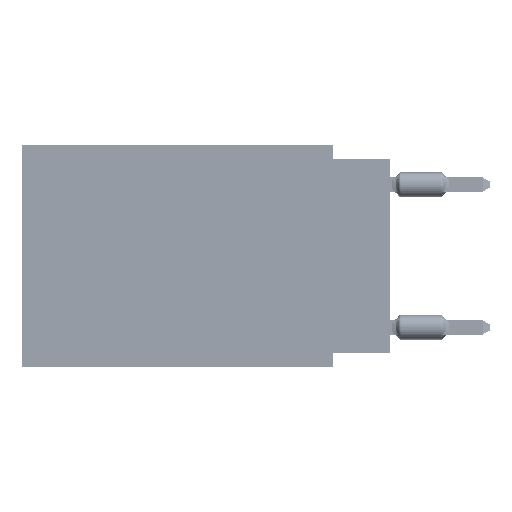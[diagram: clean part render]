
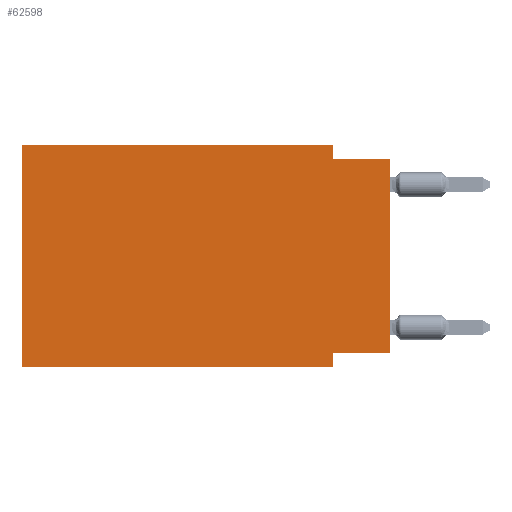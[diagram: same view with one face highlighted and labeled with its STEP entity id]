
A CAD part, left-side view. The second image highlights one B-rep face of the part: STEP entity #62598.
In plain terms, the highlighted planar face has unit normal (-1, 0, 0).
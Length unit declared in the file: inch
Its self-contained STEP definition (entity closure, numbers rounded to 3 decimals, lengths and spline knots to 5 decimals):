
#999 = LINE ( 'NONE', #45728, #61060 ) ;
#1266 = VERTEX_POINT ( 'NONE', #63140 ) ;
#2032 = PLANE ( 'NONE',  #42727 ) ;
#4770 = CARTESIAN_POINT ( 'NONE',  ( 0., 0., -0.365 ) ) ;
#6978 = CARTESIAN_POINT ( 'NONE',  ( 0., 0.1, 0. ) ) ;
#9306 = CARTESIAN_POINT ( 'NONE',  ( 0., 0.1, 0. ) ) ;
#11625 = EDGE_CURVE ( 'NONE', #47348, #21724, #61933, .T. ) ;
#12854 = CARTESIAN_POINT ( 'NONE',  ( 0., 0.645, 0. ) ) ;
#13706 = ORIENTED_EDGE ( 'NONE', *, *, #64190, .F. ) ;
#14523 = VERTEX_POINT ( 'NONE', #38025 ) ;
#15894 = CARTESIAN_POINT ( 'NONE',  ( 0., 0., -0.365 ) ) ;
#19390 = ORIENTED_EDGE ( 'NONE', *, *, #35531, .F. ) ;
#19460 = DIRECTION ( 'NONE',  ( 1., 0., 0. ) ) ;
#21682 = CARTESIAN_POINT ( 'NONE',  ( 0., 0.1, -0.39 ) ) ;
#21724 = VERTEX_POINT ( 'NONE', #50096 ) ;
#24328 = LINE ( 'NONE', #36049, #53597 ) ;
#26600 = VERTEX_POINT ( 'NONE', #57819 ) ;
#29452 = CARTESIAN_POINT ( 'NONE',  ( 0., 0., -0.025 ) ) ;
#30628 = ORIENTED_EDGE ( 'NONE', *, *, #65750, .T. ) ;
#31899 = LINE ( 'NONE', #21682, #41519 ) ;
#33977 = CARTESIAN_POINT ( 'NONE',  ( 0., 0.645, -0.39 ) ) ;
#35531 = EDGE_CURVE ( 'NONE', #26600, #1266, #31899, .T. ) ;
#35904 = VECTOR ( 'NONE', #38977, 39.37008 ) ;
#36049 = CARTESIAN_POINT ( 'NONE',  ( 0., 0.645, 0. ) ) ;
#38025 = CARTESIAN_POINT ( 'NONE',  ( 0., 0., -0.025 ) ) ;
#38471 = DIRECTION ( 'NONE',  ( 0., 0., -1. ) ) ;
#38977 = DIRECTION ( 'NONE',  ( 0., 1., 0. ) ) ;
#39335 = EDGE_CURVE ( 'NONE', #46749, #1266, #55538, .T. ) ;
#41519 = VECTOR ( 'NONE', #72012, 39.37008 ) ;
#41805 = EDGE_CURVE ( 'NONE', #60096, #26600, #62071, .T. ) ;
#42095 = DIRECTION ( 'NONE',  ( 0., -1., 0. ) ) ;
#42710 = VECTOR ( 'NONE', #38471, 39.37008 ) ;
#42727 = AXIS2_PLACEMENT_3D ( 'NONE', #71304, #19460, #65637 ) ;
#45684 = VERTEX_POINT ( 'NONE', #60747 ) ;
#45688 = DIRECTION ( 'NONE',  ( 0., -1., 0. ) ) ;
#45728 = CARTESIAN_POINT ( 'NONE',  ( 0., 0., 0. ) ) ;
#46088 = DIRECTION ( 'NONE',  ( 0., 0., 1. ) ) ;
#46221 = LINE ( 'NONE', #12854, #67586 ) ;
#46749 = VERTEX_POINT ( 'NONE', #69929 ) ;
#47348 = VERTEX_POINT ( 'NONE', #6978 ) ;
#50096 = CARTESIAN_POINT ( 'NONE',  ( 0., 0.1, -0.025 ) ) ;
#51971 = EDGE_LOOP ( 'NONE', ( #30628, #70944, #58497, #13706, #68770, #55438, #19390, #74745 ) ) ;
#52522 = DIRECTION ( 'NONE',  ( 0., -1., 0. ) ) ;
#53597 = VECTOR ( 'NONE', #42095, 39.37008 ) ;
#53895 = FACE_OUTER_BOUND ( 'NONE', #51971, .T. ) ;
#55032 = VECTOR ( 'NONE', #45688, 39.37008 ) ;
#55438 = ORIENTED_EDGE ( 'NONE', *, *, #39335, .T. ) ;
#55538 = LINE ( 'NONE', #33977, #55032 ) ;
#56800 = EDGE_CURVE ( 'NONE', #46749, #45684, #46221, .T. ) ;
#57819 = CARTESIAN_POINT ( 'NONE',  ( 0., 0.1, -0.365 ) ) ;
#58215 = LINE ( 'NONE', #29452, #72512 ) ;
#58315 = DIRECTION ( 'NONE',  ( 0., 0., 1. ) ) ;
#58497 = ORIENTED_EDGE ( 'NONE', *, *, #11625, .F. ) ;
#60096 = VERTEX_POINT ( 'NONE', #4770 ) ;
#60747 = CARTESIAN_POINT ( 'NONE',  ( 0., 0.645, 0. ) ) ;
#61060 = VECTOR ( 'NONE', #46088, 39.37008 ) ;
#61933 = LINE ( 'NONE', #9306, #42710 ) ;
#62071 = LINE ( 'NONE', #15894, #35904 ) ;
#62598 = ADVANCED_FACE ( 'NONE', ( #53895 ), #2032, .F. ) ;
#63140 = CARTESIAN_POINT ( 'NONE',  ( 0., 0.1, -0.39 ) ) ;
#64190 = EDGE_CURVE ( 'NONE', #45684, #47348, #24328, .T. ) ;
#65637 = DIRECTION ( 'NONE',  ( 0., 0., -1. ) ) ;
#65750 = EDGE_CURVE ( 'NONE', #60096, #14523, #999, .T. ) ;
#67586 = VECTOR ( 'NONE', #58315, 39.37008 ) ;
#68770 = ORIENTED_EDGE ( 'NONE', *, *, #56800, .F. ) ;
#69929 = CARTESIAN_POINT ( 'NONE',  ( 0., 0.645, -0.39 ) ) ;
#70944 = ORIENTED_EDGE ( 'NONE', *, *, #73254, .F. ) ;
#71304 = CARTESIAN_POINT ( 'NONE',  ( 0., 0.645, 0. ) ) ;
#72012 = DIRECTION ( 'NONE',  ( 0., 0., -1. ) ) ;
#72512 = VECTOR ( 'NONE', #52522, 39.37008 ) ;
#73254 = EDGE_CURVE ( 'NONE', #21724, #14523, #58215, .T. ) ;
#74745 = ORIENTED_EDGE ( 'NONE', *, *, #41805, .F. ) ;
